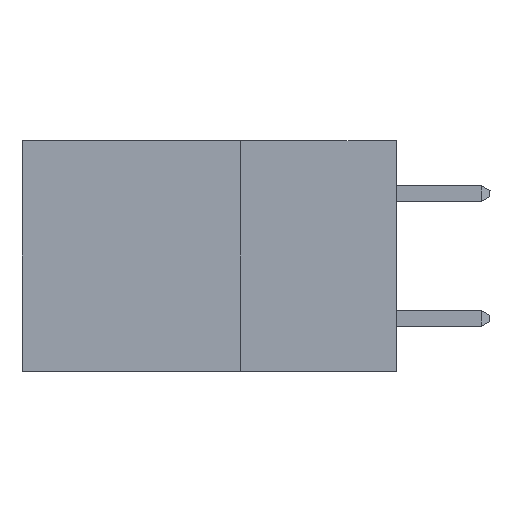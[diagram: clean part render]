
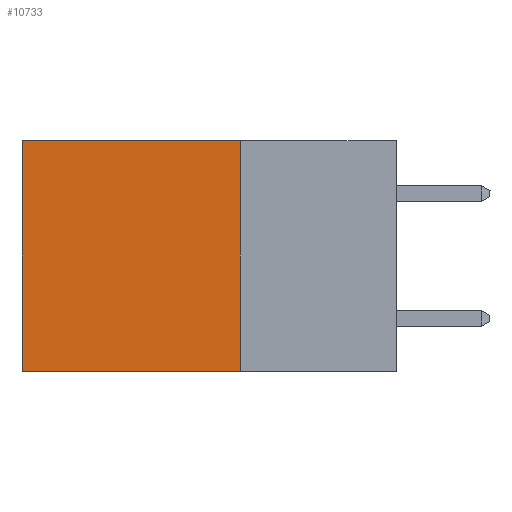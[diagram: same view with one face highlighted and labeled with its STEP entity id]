
A CAD part, left-side view. The second image highlights one B-rep face of the part: STEP entity #10733.
In plain terms, the highlighted planar face has unit normal (-1, 0, 0).
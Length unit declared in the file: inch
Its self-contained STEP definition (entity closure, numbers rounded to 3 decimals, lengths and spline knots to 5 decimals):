
#669 = CARTESIAN_POINT ( 'NONE',  ( 0.298, 0.6, 0. ) ) ;
#960 = EDGE_CURVE ( 'NONE', #3319, #6998, #2854, .T. ) ;
#1075 = ORIENTED_EDGE ( 'NONE', *, *, #10496, .F. ) ;
#1252 = AXIS2_PLACEMENT_3D ( 'NONE', #16639, #12914, #4995 ) ;
#1333 = CARTESIAN_POINT ( 'NONE',  ( 0.298, 0.25, 0. ) ) ;
#2087 = CARTESIAN_POINT ( 'NONE',  ( 0.298, 0.6, 0. ) ) ;
#2427 = LINE ( 'NONE', #8015, #5618 ) ;
#2793 = LINE ( 'NONE', #16259, #6378 ) ;
#2854 = LINE ( 'NONE', #669, #6017 ) ;
#3319 = VERTEX_POINT ( 'NONE', #2087 ) ;
#3364 = LINE ( 'NONE', #4345, #13496 ) ;
#3642 = PLANE ( 'NONE',  #1252 ) ;
#4345 = CARTESIAN_POINT ( 'NONE',  ( 0.298, 0.25, -0.37 ) ) ;
#4485 = DIRECTION ( 'NONE',  ( 0., 0., -1. ) ) ;
#4995 = DIRECTION ( 'NONE',  ( 0., 0., -1. ) ) ;
#5618 = VECTOR ( 'NONE', #6722, 39.37008 ) ;
#5760 = FACE_OUTER_BOUND ( 'NONE', #7011, .T. ) ;
#6017 = VECTOR ( 'NONE', #7660, 39.37008 ) ;
#6378 = VECTOR ( 'NONE', #4485, 39.37008 ) ;
#6722 = DIRECTION ( 'NONE',  ( 0., 1., 0. ) ) ;
#6998 = VERTEX_POINT ( 'NONE', #13152 ) ;
#7011 = EDGE_LOOP ( 'NONE', ( #16689, #15417, #1075, #12802 ) ) ;
#7660 = DIRECTION ( 'NONE',  ( 0., 0., -1. ) ) ;
#8015 = CARTESIAN_POINT ( 'NONE',  ( 0.298, 0.25, 0. ) ) ;
#9689 = VERTEX_POINT ( 'NONE', #12660 ) ;
#10496 = EDGE_CURVE ( 'NONE', #13114, #9689, #2793, .T. ) ;
#10733 = ADVANCED_FACE ( 'NONE', ( #5760 ), #3642, .F. ) ;
#11008 = DIRECTION ( 'NONE',  ( 0., 1., 0. ) ) ;
#12660 = CARTESIAN_POINT ( 'NONE',  ( 0.298, 0.25, -0.37 ) ) ;
#12802 = ORIENTED_EDGE ( 'NONE', *, *, #16473, .T. ) ;
#12914 = DIRECTION ( 'NONE',  ( 1., 0., 0. ) ) ;
#13114 = VERTEX_POINT ( 'NONE', #1333 ) ;
#13152 = CARTESIAN_POINT ( 'NONE',  ( 0.298, 0.6, -0.37 ) ) ;
#13496 = VECTOR ( 'NONE', #11008, 39.37008 ) ;
#14320 = EDGE_CURVE ( 'NONE', #9689, #6998, #3364, .T. ) ;
#15417 = ORIENTED_EDGE ( 'NONE', *, *, #14320, .F. ) ;
#16259 = CARTESIAN_POINT ( 'NONE',  ( 0.298, 0.25, 0. ) ) ;
#16473 = EDGE_CURVE ( 'NONE', #13114, #3319, #2427, .T. ) ;
#16639 = CARTESIAN_POINT ( 'NONE',  ( 0.298, 0.25, 0. ) ) ;
#16689 = ORIENTED_EDGE ( 'NONE', *, *, #960, .T. ) ;
